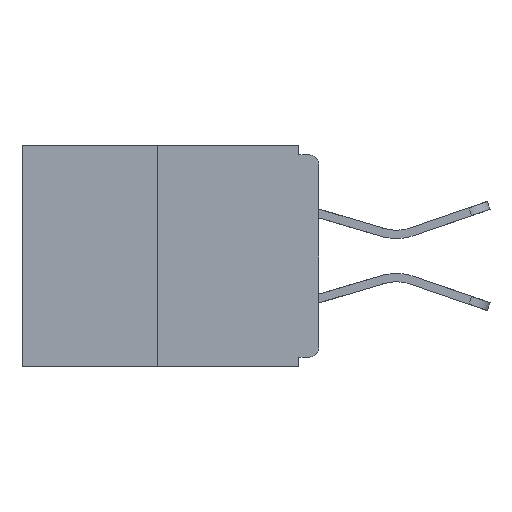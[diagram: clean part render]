
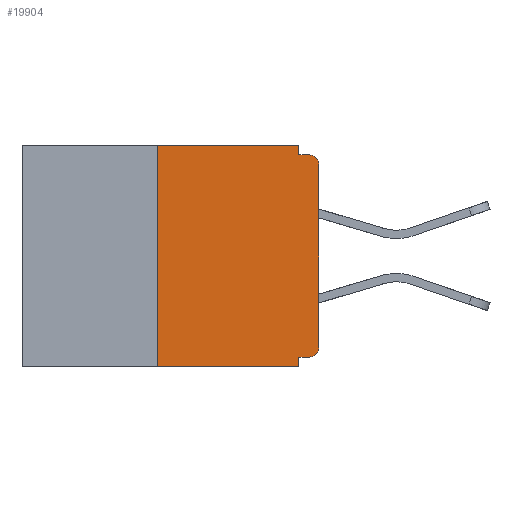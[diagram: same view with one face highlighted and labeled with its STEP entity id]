
A CAD part, left-side view. The second image highlights one B-rep face of the part: STEP entity #19904.
In plain terms, the highlighted planar face has unit normal (-1, 0, 0).
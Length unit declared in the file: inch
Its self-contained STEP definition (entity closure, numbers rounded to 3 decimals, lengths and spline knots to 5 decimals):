
#26 = LINE ( 'NONE', #7311, #13609 ) ;
#192 = EDGE_CURVE ( 'NONE', #18529, #13066, #8996, .T. ) ;
#263 = EDGE_CURVE ( 'NONE', #15265, #12092, #23220, .T. ) ;
#266 = DIRECTION ( 'NONE',  ( 0., -1., 0. ) ) ;
#525 = CARTESIAN_POINT ( 'NONE',  ( 0., 0.015, -0.328 ) ) ;
#592 = VERTEX_POINT ( 'NONE', #17743 ) ;
#913 = CARTESIAN_POINT ( 'NONE',  ( 0., 0.015, -0.313 ) ) ;
#991 = CARTESIAN_POINT ( 'NONE',  ( 0., 0., 0. ) ) ;
#1130 = DIRECTION ( 'NONE',  ( -1., 0., 0. ) ) ;
#1763 = CARTESIAN_POINT ( 'NONE',  ( 0., 0.031, 0. ) ) ;
#2278 = LINE ( 'NONE', #16545, #7475 ) ;
#2328 = CARTESIAN_POINT ( 'NONE',  ( 0., 0.46, -0.343 ) ) ;
#2341 = VERTEX_POINT ( 'NONE', #525 ) ;
#2657 = LINE ( 'NONE', #20377, #9571 ) ;
#2693 = DIRECTION ( 'NONE',  ( 0., 0., -1. ) ) ;
#2937 = DIRECTION ( 'NONE',  ( 0., 0., 1. ) ) ;
#3343 = DIRECTION ( 'NONE',  ( 0., -1., 0. ) ) ;
#3373 = AXIS2_PLACEMENT_3D ( 'NONE', #913, #13740, #2693 ) ;
#3690 = EDGE_LOOP ( 'NONE', ( #18007, #7219, #23232, #18946, #9356, #17146, #17522, #6965, #13192, #6626 ) ) ;
#3722 = CARTESIAN_POINT ( 'NONE',  ( 0., 0., -0.015 ) ) ;
#3771 = VERTEX_POINT ( 'NONE', #12160 ) ;
#4161 = EDGE_CURVE ( 'NONE', #592, #15265, #26, .T. ) ;
#4332 = LINE ( 'NONE', #3722, #17932 ) ;
#4382 = AXIS2_PLACEMENT_3D ( 'NONE', #21770, #23620, #12471 ) ;
#4486 = VERTEX_POINT ( 'NONE', #19705 ) ;
#5855 = EDGE_CURVE ( 'NONE', #12092, #13066, #4332, .T. ) ;
#6573 = CARTESIAN_POINT ( 'NONE',  ( 0., 0., -0.03 ) ) ;
#6626 = ORIENTED_EDGE ( 'NONE', *, *, #263, .F. ) ;
#6965 = ORIENTED_EDGE ( 'NONE', *, *, #192, .T. ) ;
#7219 = ORIENTED_EDGE ( 'NONE', *, *, #12519, .F. ) ;
#7311 = CARTESIAN_POINT ( 'NONE',  ( 0., 0.46, 0. ) ) ;
#7418 = LINE ( 'NONE', #2328, #9742 ) ;
#7475 = VECTOR ( 'NONE', #20499, 39.37008 ) ;
#7538 = LINE ( 'NONE', #991, #9552 ) ;
#8996 = CIRCLE ( 'NONE', #10775, 0.015 ) ;
#9356 = ORIENTED_EDGE ( 'NONE', *, *, #18031, .F. ) ;
#9552 = VECTOR ( 'NONE', #2937, 39.37008 ) ;
#9571 = VECTOR ( 'NONE', #11279, 39.37008 ) ;
#9742 = VECTOR ( 'NONE', #11680, 39.37008 ) ;
#9768 = DIRECTION ( 'NONE',  ( 0., 0., -1. ) ) ;
#10775 = AXIS2_PLACEMENT_3D ( 'NONE', #21721, #1130, #23406 ) ;
#11279 = DIRECTION ( 'NONE',  ( 0., 1., 0. ) ) ;
#11580 = VECTOR ( 'NONE', #9768, 39.37008 ) ;
#11680 = DIRECTION ( 'NONE',  ( 0., -1., 0. ) ) ;
#11869 = CARTESIAN_POINT ( 'NONE',  ( 0., 0.015, -0.015 ) ) ;
#12092 = VERTEX_POINT ( 'NONE', #21881 ) ;
#12160 = CARTESIAN_POINT ( 'NONE',  ( 0., 0.031, -0.343 ) ) ;
#12344 = EDGE_CURVE ( 'NONE', #4486, #3771, #7418, .T. ) ;
#12471 = DIRECTION ( 'NONE',  ( 0., 0., -1. ) ) ;
#12519 = EDGE_CURVE ( 'NONE', #4486, #592, #21957, .T. ) ;
#13066 = VERTEX_POINT ( 'NONE', #11869 ) ;
#13192 = ORIENTED_EDGE ( 'NONE', *, *, #5855, .F. ) ;
#13484 = VECTOR ( 'NONE', #17533, 39.37008 ) ;
#13609 = VECTOR ( 'NONE', #3343, 39.37008 ) ;
#13740 = DIRECTION ( 'NONE',  ( -1., 0., 0. ) ) ;
#13869 = CARTESIAN_POINT ( 'NONE',  ( 0., 0.031, 0. ) ) ;
#14042 = EDGE_CURVE ( 'NONE', #21756, #3771, #2278, .T. ) ;
#14270 = CARTESIAN_POINT ( 'NONE',  ( 0., 0.031, -0.328 ) ) ;
#14603 = EDGE_CURVE ( 'NONE', #2341, #22594, #20187, .T. ) ;
#15265 = VERTEX_POINT ( 'NONE', #13869 ) ;
#16545 = CARTESIAN_POINT ( 'NONE',  ( 0., 0.031, -0.343 ) ) ;
#17146 = ORIENTED_EDGE ( 'NONE', *, *, #14603, .T. ) ;
#17522 = ORIENTED_EDGE ( 'NONE', *, *, #19238, .T. ) ;
#17533 = DIRECTION ( 'NONE',  ( 0., 0., 1. ) ) ;
#17743 = CARTESIAN_POINT ( 'NONE',  ( 0., 0.25, 0. ) ) ;
#17932 = VECTOR ( 'NONE', #266, 39.37008 ) ;
#18007 = ORIENTED_EDGE ( 'NONE', *, *, #4161, .F. ) ;
#18031 = EDGE_CURVE ( 'NONE', #2341, #21756, #2657, .T. ) ;
#18529 = VERTEX_POINT ( 'NONE', #6573 ) ;
#18946 = ORIENTED_EDGE ( 'NONE', *, *, #14042, .F. ) ;
#19238 = EDGE_CURVE ( 'NONE', #22594, #18529, #7538, .T. ) ;
#19319 = CARTESIAN_POINT ( 'NONE',  ( 0., 0.25, 0. ) ) ;
#19705 = CARTESIAN_POINT ( 'NONE',  ( 0., 0.25, -0.343 ) ) ;
#19892 = FACE_OUTER_BOUND ( 'NONE', #3690, .T. ) ;
#19904 = ADVANCED_FACE ( 'NONE', ( #19892 ), #21614, .F. ) ;
#20187 = CIRCLE ( 'NONE', #3373, 0.015 ) ;
#20377 = CARTESIAN_POINT ( 'NONE',  ( 0., 0., -0.328 ) ) ;
#20499 = DIRECTION ( 'NONE',  ( 0., 0., -1. ) ) ;
#20756 = CARTESIAN_POINT ( 'NONE',  ( 0., 0., -0.313 ) ) ;
#21614 = PLANE ( 'NONE',  #4382 ) ;
#21721 = CARTESIAN_POINT ( 'NONE',  ( 0., 0.015, -0.03 ) ) ;
#21756 = VERTEX_POINT ( 'NONE', #14270 ) ;
#21770 = CARTESIAN_POINT ( 'NONE',  ( 0., 0.46, 0. ) ) ;
#21881 = CARTESIAN_POINT ( 'NONE',  ( 0., 0.031, -0.015 ) ) ;
#21957 = LINE ( 'NONE', #19319, #13484 ) ;
#22594 = VERTEX_POINT ( 'NONE', #20756 ) ;
#23220 = LINE ( 'NONE', #1763, #11580 ) ;
#23232 = ORIENTED_EDGE ( 'NONE', *, *, #12344, .T. ) ;
#23406 = DIRECTION ( 'NONE',  ( 0., 0., -1. ) ) ;
#23620 = DIRECTION ( 'NONE',  ( 1., 0., 0. ) ) ;
